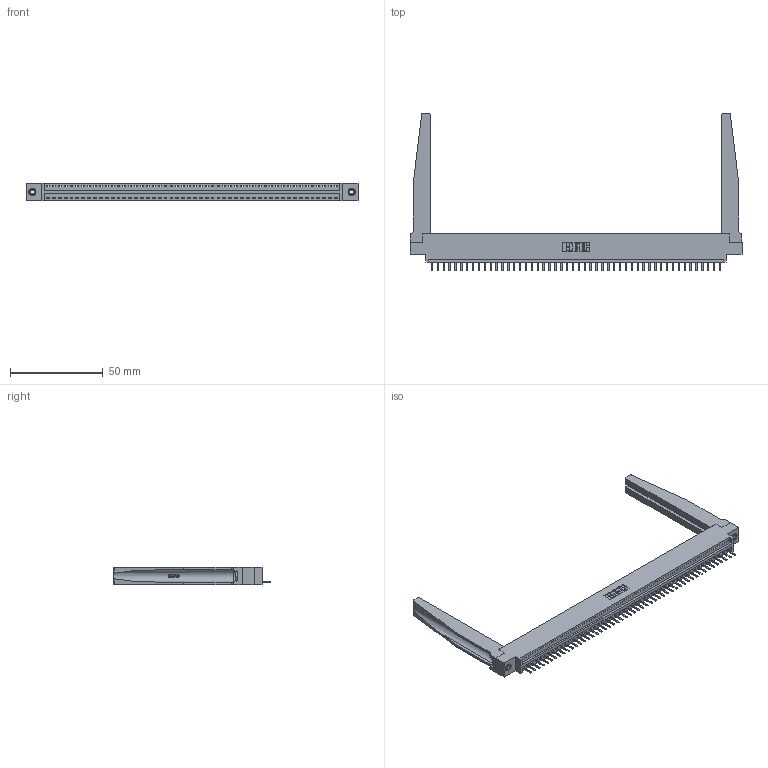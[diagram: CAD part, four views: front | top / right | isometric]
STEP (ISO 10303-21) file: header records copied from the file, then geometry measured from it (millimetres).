
FILE_DESCRIPTION (( 'STEP AP203' ), '1' );
FILE_NAME ('396-050-520-678.STEP', '2019-10-28T06:05:13', ( '' ), ( '' ), 'SwSTEP 2.0', 'SolidWorks 2016', '' );
FILE_SCHEMA (( 'CONFIG_CONTROL_DESIGN' ));
Length unit declared in the file: inch
Products named in the file (5): 345-292-001_345-293-120; 346 Part_0.170 Offset - 0.156 Dia-TH; 346-220-078_345-220-078; 345-250-001_345-250-001-102; 396-050-520-678
Assembly tree (55 placements, depth 2):
  396-050-520-678
    346 Part_0.170 Offset - 0.156 Dia-TH
    345-292-001_345-293-120  x50
    346-220-078_345-220-078  x2
    345-250-001_345-250-001-102  x2
Bounding box: 179.32 x 85.29 x 9.4 mm (x, y, z)
Volume: 23830.8 mm3; surface area: 27456.9 mm2
Topology: 55 solids, 55 shells, 3460 faces, 10149 edges, 6622 vertices
Faces by surface type: plane 2322, cylinder 1086, bspline 36, cone 12, torus 4
Entity records: 34948 total; most frequent: CARTESIAN_POINT 6913, ORIENTED_EDGE 5774, DIRECTION 5061, EDGE_CURVE 2887, LINE 2457, VECTOR 2457, VERTEX_POINT 1916, AXIS2_PLACEMENT_3D 1302
